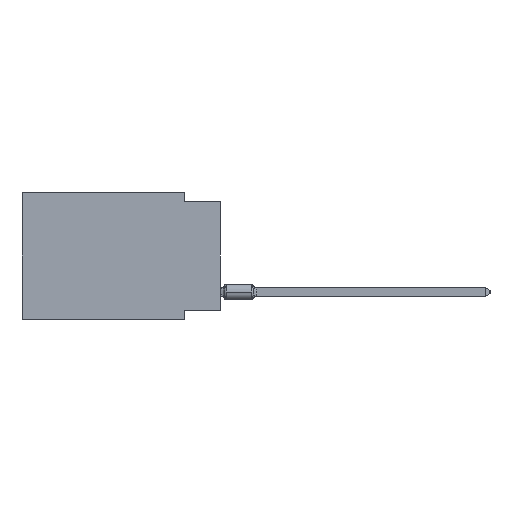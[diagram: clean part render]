
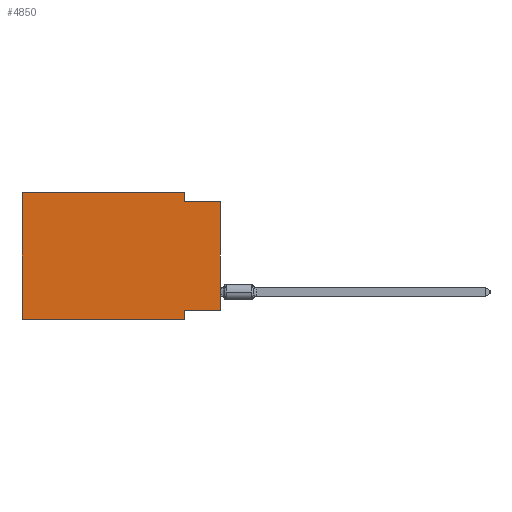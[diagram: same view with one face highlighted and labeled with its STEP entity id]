
A CAD part, left-side view. The second image highlights one B-rep face of the part: STEP entity #4850.
In plain terms, the highlighted planar face has unit normal (-1, 0, 0).
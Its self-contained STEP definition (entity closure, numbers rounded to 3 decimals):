
#294 = LINE ( 'NONE', #4994, #14022 ) ;
#343 = VERTEX_POINT ( 'NONE', #22674 ) ;
#366 = VECTOR ( 'NONE', #7780, 1000. ) ;
#789 = CARTESIAN_POINT ( 'NONE',  ( 0., 13.97, 0. ) ) ;
#1201 = ORIENTED_EDGE ( 'NONE', *, *, #14372, .F. ) ;
#1444 = EDGE_CURVE ( 'NONE', #16404, #13119, #294, .T. ) ;
#2439 = LINE ( 'NONE', #7827, #15538 ) ;
#3123 = VECTOR ( 'NONE', #4422, 1000. ) ;
#3154 = DIRECTION ( 'NONE',  ( 0., 0., -1. ) ) ;
#3615 = EDGE_CURVE ( 'NONE', #14465, #6968, #21086, .T. ) ;
#3775 = LINE ( 'NONE', #20791, #22025 ) ;
#3792 = CARTESIAN_POINT ( 'NONE',  ( 0., 0., -0.635 ) ) ;
#3825 = VECTOR ( 'NONE', #19580, 1000. ) ;
#4422 = DIRECTION ( 'NONE',  ( 0., 0., -1. ) ) ;
#4593 = CARTESIAN_POINT ( 'NONE',  ( 0., 13.97, -8.89 ) ) ;
#4806 = LINE ( 'NONE', #20425, #18939 ) ;
#4850 = ADVANCED_FACE ( 'NONE', ( #7176 ), #12445, .F. ) ;
#4994 = CARTESIAN_POINT ( 'NONE',  ( 0., 2.54, 0. ) ) ;
#5182 = ORIENTED_EDGE ( 'NONE', *, *, #3615, .F. ) ;
#5351 = CARTESIAN_POINT ( 'NONE',  ( 0., 0., -8.255 ) ) ;
#5766 = VECTOR ( 'NONE', #22611, 1000. ) ;
#6595 = CARTESIAN_POINT ( 'NONE',  ( 0., 13.97, 0. ) ) ;
#6968 = VERTEX_POINT ( 'NONE', #18323 ) ;
#7176 = FACE_OUTER_BOUND ( 'NONE', #11362, .T. ) ;
#7780 = DIRECTION ( 'NONE',  ( 0., -1., 0. ) ) ;
#7827 = CARTESIAN_POINT ( 'NONE',  ( 0., 13.97, 0. ) ) ;
#7860 = VERTEX_POINT ( 'NONE', #6595 ) ;
#8032 = CARTESIAN_POINT ( 'NONE',  ( 0., 0., -8.255 ) ) ;
#9566 = DIRECTION ( 'NONE',  ( 0., 0., 1. ) ) ;
#9761 = ORIENTED_EDGE ( 'NONE', *, *, #12546, .F. ) ;
#10493 = ORIENTED_EDGE ( 'NONE', *, *, #1444, .F. ) ;
#11116 = LINE ( 'NONE', #789, #366 ) ;
#11278 = VERTEX_POINT ( 'NONE', #4593 ) ;
#11362 = EDGE_LOOP ( 'NONE', ( #12732, #1201, #10493, #11682, #19153, #17142, #9761, #5182 ) ) ;
#11682 = ORIENTED_EDGE ( 'NONE', *, *, #19149, .F. ) ;
#12115 = DIRECTION ( 'NONE',  ( 0., 0., -1. ) ) ;
#12445 = PLANE ( 'NONE',  #13367 ) ;
#12546 = EDGE_CURVE ( 'NONE', #6968, #343, #20157, .T. ) ;
#12732 = ORIENTED_EDGE ( 'NONE', *, *, #14583, .T. ) ;
#13119 = VERTEX_POINT ( 'NONE', #19175 ) ;
#13367 = AXIS2_PLACEMENT_3D ( 'NONE', #14171, #22676, #3154 ) ;
#14022 = VECTOR ( 'NONE', #12115, 1000. ) ;
#14038 = VERTEX_POINT ( 'NONE', #3792 ) ;
#14105 = LINE ( 'NONE', #15594, #5766 ) ;
#14171 = CARTESIAN_POINT ( 'NONE',  ( 0., 13.97, 0. ) ) ;
#14372 = EDGE_CURVE ( 'NONE', #13119, #14038, #4806, .T. ) ;
#14465 = VERTEX_POINT ( 'NONE', #8032 ) ;
#14583 = EDGE_CURVE ( 'NONE', #14465, #14038, #14105, .T. ) ;
#15538 = VECTOR ( 'NONE', #9566, 1000. ) ;
#15594 = CARTESIAN_POINT ( 'NONE',  ( 0., 0., 0. ) ) ;
#16404 = VERTEX_POINT ( 'NONE', #16706 ) ;
#16706 = CARTESIAN_POINT ( 'NONE',  ( 0., 2.54, 0. ) ) ;
#16717 = CARTESIAN_POINT ( 'NONE',  ( 0., 2.54, -8.89 ) ) ;
#17142 = ORIENTED_EDGE ( 'NONE', *, *, #19946, .T. ) ;
#17764 = DIRECTION ( 'NONE',  ( 0., -1., 0. ) ) ;
#18323 = CARTESIAN_POINT ( 'NONE',  ( 0., 2.54, -8.255 ) ) ;
#18915 = DIRECTION ( 'NONE',  ( 0., -1., 0. ) ) ;
#18939 = VECTOR ( 'NONE', #18915, 1000. ) ;
#19149 = EDGE_CURVE ( 'NONE', #7860, #16404, #11116, .T. ) ;
#19153 = ORIENTED_EDGE ( 'NONE', *, *, #22626, .F. ) ;
#19175 = CARTESIAN_POINT ( 'NONE',  ( 0., 2.54, -0.635 ) ) ;
#19580 = DIRECTION ( 'NONE',  ( 0., 1., 0. ) ) ;
#19946 = EDGE_CURVE ( 'NONE', #11278, #343, #3775, .T. ) ;
#20157 = LINE ( 'NONE', #16717, #3123 ) ;
#20425 = CARTESIAN_POINT ( 'NONE',  ( 0., 0., -0.635 ) ) ;
#20791 = CARTESIAN_POINT ( 'NONE',  ( 0., 13.97, -8.89 ) ) ;
#21086 = LINE ( 'NONE', #5351, #3825 ) ;
#22025 = VECTOR ( 'NONE', #17764, 1000. ) ;
#22611 = DIRECTION ( 'NONE',  ( 0., 0., 1. ) ) ;
#22626 = EDGE_CURVE ( 'NONE', #11278, #7860, #2439, .T. ) ;
#22674 = CARTESIAN_POINT ( 'NONE',  ( 0., 2.54, -8.89 ) ) ;
#22676 = DIRECTION ( 'NONE',  ( 1., 0., 0. ) ) ;
